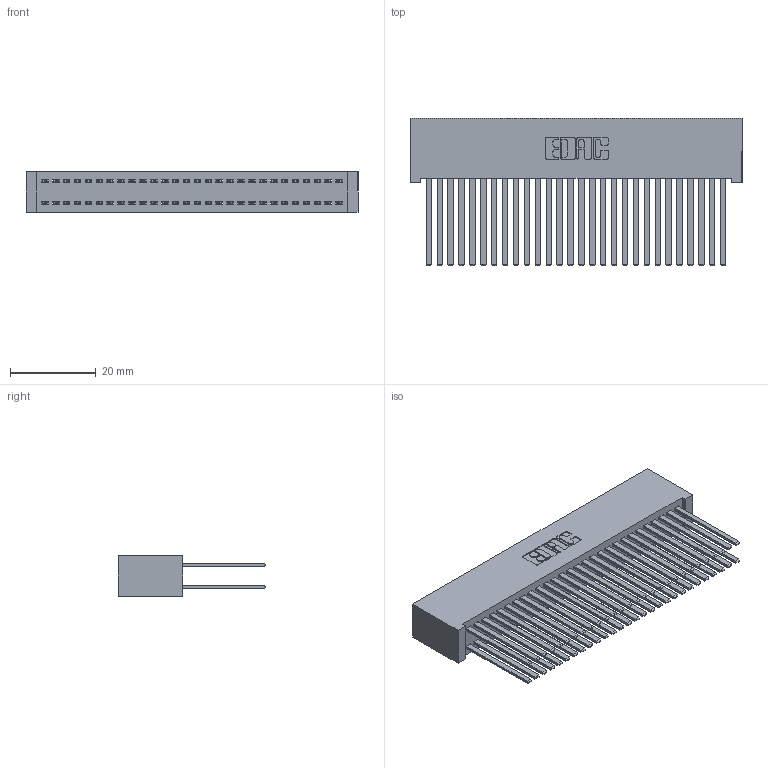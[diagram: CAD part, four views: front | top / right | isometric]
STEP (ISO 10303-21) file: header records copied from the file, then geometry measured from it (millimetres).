
FILE_DESCRIPTION (( 'STEP AP203' ), '1' );
FILE_NAME ('392-056-544-201.STEP', '2018-08-17T13:35:02', ( '' ), ( '' ), 'SwSTEP 2.0', 'SolidWorks 2016', '' );
FILE_SCHEMA (( 'CONFIG_CONTROL_DESIGN' ));
Length unit declared in the file: inch
Products named in the file (3): 342 Part_Lugless; 345-292-001_345-293-144; 392-056-544-201
Assembly tree (57 placements, depth 2):
  392-056-544-201
    342 Part_Lugless
    345-292-001_345-293-144  x56
Bounding box: 77.37 x 34.3 x 9.4 mm (x, y, z)
Volume: 8109.8 mm3; surface area: 15476 mm2
Topology: 57 solids, 57 shells, 2678 faces, 7947 edges, 5222 vertices
Faces by surface type: plane 1854, cylinder 824
Entity records: 19231 total; most frequent: CARTESIAN_POINT 3198, ORIENTED_EDGE 3134, DIRECTION 2747, EDGE_CURVE 1567, LINE 1451, VECTOR 1451, VERTEX_POINT 1042, AXIS2_PLACEMENT_3D 648
